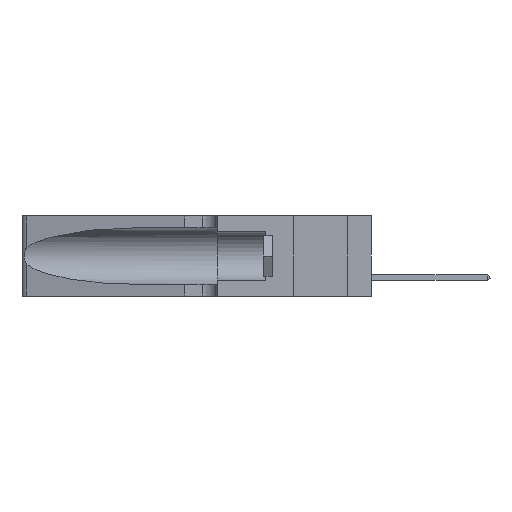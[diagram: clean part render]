
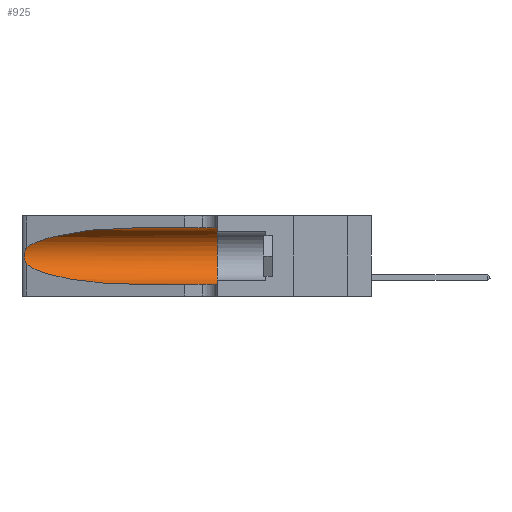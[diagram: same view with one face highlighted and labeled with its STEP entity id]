
A CAD part, left-side view. The second image highlights one B-rep face of the part: STEP entity #925.
In plain terms, the highlighted cylindrical face has radius 3.308 mm (diameter 6.617 mm), a partial arc.
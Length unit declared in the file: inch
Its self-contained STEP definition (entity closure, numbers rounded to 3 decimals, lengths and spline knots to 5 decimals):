
#410 = CARTESIAN_POINT ( 'NONE',  ( 0.18966, 0.96281, 0.31525 ) ) ;
#536 = AXIS2_PLACEMENT_3D ( 'NONE', #7826, #24264, #11922 ) ;
#689 = CARTESIAN_POINT ( 'NONE',  ( 0.1305, 1.61858, 0.31525 ) ) ;
#870 = CARTESIAN_POINT ( 'NONE',  ( 0.25487, 1.22718, 0.22369 ) ) ;
#925 = ADVANCED_FACE ( 'NONE', ( #7799 ), #13868, .F. ) ;
#1193 = CARTESIAN_POINT ( 'NONE',  ( 0.1305, 1.61858, 0.185 ) ) ;
#1276 = CARTESIAN_POINT ( 'NONE',  ( 0.25856, 1.23593, 0.16098 ) ) ;
#1287 =( BOUNDED_CURVE ( )  B_SPLINE_CURVE ( 3, ( #19634, #5192, #23775, #15300 ),
 .UNSPECIFIED., .F., .T. ) 
 B_SPLINE_CURVE_WITH_KNOTS ( ( 4, 4 ),
 ( 3.44316, 4.71239 ),
 .UNSPECIFIED. ) 
 CURVE ( )  GEOMETRIC_REPRESENTATION_ITEM ( )  RATIONAL_B_SPLINE_CURVE ( ( 1., 0.87, 0.87, 1. ) ) 
 REPRESENTATION_ITEM ( '' )  );
#1409 = DIRECTION ( 'NONE',  ( 0., -1., 0. ) ) ;
#2575 = CARTESIAN_POINT ( 'NONE',  ( 0.1305, 0.72297, 0.31525 ) ) ;
#3420 = VERTEX_POINT ( 'NONE', #14560 ) ;
#3459 = ORIENTED_EDGE ( 'NONE', *, *, #3870, .T. ) ;
#3516 = CARTESIAN_POINT ( 'NONE',  ( 0.25789, 1.23486, 0.15765 ) ) ;
#3870 = EDGE_CURVE ( 'NONE', #22894, #8590, #14349, .T. ) ;
#4052 = DIRECTION ( 'NONE',  ( 0., 0., -1. ) ) ;
#4432 = CARTESIAN_POINT ( 'NONE',  ( 0.25487, 1.22718, 0.22369 ) ) ;
#4569 = AXIS2_PLACEMENT_3D ( 'NONE', #1193, #21675, #4052 ) ;
#4648 = CARTESIAN_POINT ( 'NONE',  ( 0.1305, 0.35, 0.31525 ) ) ;
#5192 = CARTESIAN_POINT ( 'NONE',  ( 0.2373, 1.15595, 0.08982 ) ) ;
#6901 = EDGE_CURVE ( 'NONE', #12068, #13662, #10898, .T. ) ;
#7421 = CARTESIAN_POINT ( 'NONE',  ( 0.25639, 1.23186, 0.15144 ) ) ;
#7693 = CARTESIAN_POINT ( 'NONE',  ( 0.26017, 1.23833, 0.17102 ) ) ;
#7799 = FACE_OUTER_BOUND ( 'NONE', #14901, .T. ) ;
#7826 = CARTESIAN_POINT ( 'NONE',  ( 0.1305, 0.35, 0.185 ) ) ;
#8590 = VERTEX_POINT ( 'NONE', #870 ) ;
#9244 = ORIENTED_EDGE ( 'NONE', *, *, #19652, .T. ) ;
#9536 = ORIENTED_EDGE ( 'NONE', *, *, #20752, .T. ) ;
#10898 = CIRCLE ( 'NONE', #536, 0.13025 ) ;
#11234 = CARTESIAN_POINT ( 'NONE',  ( 0.25487, 1.22718, 0.14631 ) ) ;
#11513 = CARTESIAN_POINT ( 'NONE',  ( 0.26018, 1.23835, 0.19895 ) ) ;
#11625 = ORIENTED_EDGE ( 'NONE', *, *, #24543, .T. ) ;
#11922 = DIRECTION ( 'NONE',  ( 0., 0., 1. ) ) ;
#12068 = VERTEX_POINT ( 'NONE', #4648 ) ;
#13580 = CARTESIAN_POINT ( 'NONE',  ( 0.25555, 1.22993, 0.14849 ) ) ;
#13662 = VERTEX_POINT ( 'NONE', #18364 ) ;
#13673 = CARTESIAN_POINT ( 'NONE',  ( 0.25487, 1.22718, 0.14631 ) ) ;
#13868 = CYLINDRICAL_SURFACE ( 'NONE', #4569, 0.13025 ) ;
#13932 = LINE ( 'NONE', #19955, #16759 ) ;
#14100 = CARTESIAN_POINT ( 'NONE',  ( 0.1305, 0.72297, 0.31525 ) ) ;
#14349 =( BOUNDED_CURVE ( )  B_SPLINE_CURVE ( 3, ( #2575, #410, #16642, #4432 ),
 .UNSPECIFIED., .F., .F. ) 
 B_SPLINE_CURVE_WITH_KNOTS ( ( 4, 4 ),
 ( 1.5708, 2.84003 ),
 .UNSPECIFIED. ) 
 CURVE ( )  GEOMETRIC_REPRESENTATION_ITEM ( )  RATIONAL_B_SPLINE_CURVE ( ( 1., 0.87, 0.87, 1. ) ) 
 REPRESENTATION_ITEM ( '' )  );
#14560 = CARTESIAN_POINT ( 'NONE',  ( 0.1305, 0.72297, 0.05475 ) ) ;
#14865 = B_SPLINE_CURVE_WITH_KNOTS ( 'NONE', 3,
 ( #23679, #15745, #23868, #15823, #19994, #11513, #25881, #17599, #7693, #1276, #3516, #7421, #13580, #13673 ),
 .UNSPECIFIED., .F., .F.,
 ( 4, 2, 2, 2, 2, 2, 4 ),
 ( 0., 0.00027, 0.00053, 0.00107, 0.0016, 0.00187, 0.00214 ),
 .UNSPECIFIED. ) ;
#14901 = EDGE_LOOP ( 'NONE', ( #3459, #11625, #9244, #9536, #25536, #17864 ) ) ;
#15267 = EDGE_CURVE ( 'NONE', #22894, #12068, #16097, .T. ) ;
#15300 = CARTESIAN_POINT ( 'NONE',  ( 0.1305, 0.72297, 0.05475 ) ) ;
#15745 = CARTESIAN_POINT ( 'NONE',  ( 0.25555, 1.22994, 0.2215 ) ) ;
#15823 = CARTESIAN_POINT ( 'NONE',  ( 0.25787, 1.23484, 0.2124 ) ) ;
#16097 = LINE ( 'NONE', #689, #17405 ) ;
#16642 = CARTESIAN_POINT ( 'NONE',  ( 0.2373, 1.15595, 0.28018 ) ) ;
#16759 = VECTOR ( 'NONE', #1409, 39.37008 ) ;
#17405 = VECTOR ( 'NONE', #23006, 39.37008 ) ;
#17599 = CARTESIAN_POINT ( 'NONE',  ( 0.26075, 1.23896, 0.178 ) ) ;
#17864 = ORIENTED_EDGE ( 'NONE', *, *, #15267, .F. ) ;
#18364 = CARTESIAN_POINT ( 'NONE',  ( 0.1305, 0.35, 0.05475 ) ) ;
#19634 = CARTESIAN_POINT ( 'NONE',  ( 0.25487, 1.22718, 0.14631 ) ) ;
#19645 = VERTEX_POINT ( 'NONE', #11234 ) ;
#19652 = EDGE_CURVE ( 'NONE', #19645, #3420, #1287, .T. ) ;
#19955 = CARTESIAN_POINT ( 'NONE',  ( 0.1305, 1.61858, 0.05475 ) ) ;
#19994 = CARTESIAN_POINT ( 'NONE',  ( 0.25854, 1.2359, 0.20912 ) ) ;
#20752 = EDGE_CURVE ( 'NONE', #3420, #13662, #13932, .T. ) ;
#21675 = DIRECTION ( 'NONE',  ( 0., -1., 0. ) ) ;
#22894 = VERTEX_POINT ( 'NONE', #14100 ) ;
#23006 = DIRECTION ( 'NONE',  ( 0., -1., 0. ) ) ;
#23679 = CARTESIAN_POINT ( 'NONE',  ( 0.25487, 1.22718, 0.22369 ) ) ;
#23775 = CARTESIAN_POINT ( 'NONE',  ( 0.18966, 0.96281, 0.05475 ) ) ;
#23868 = CARTESIAN_POINT ( 'NONE',  ( 0.25639, 1.23184, 0.21858 ) ) ;
#24264 = DIRECTION ( 'NONE',  ( 0., 1., 0. ) ) ;
#24543 = EDGE_CURVE ( 'NONE', #8590, #19645, #14865, .T. ) ;
#25536 = ORIENTED_EDGE ( 'NONE', *, *, #6901, .F. ) ;
#25881 = CARTESIAN_POINT ( 'NONE',  ( 0.26075, 1.23896, 0.19203 ) ) ;
